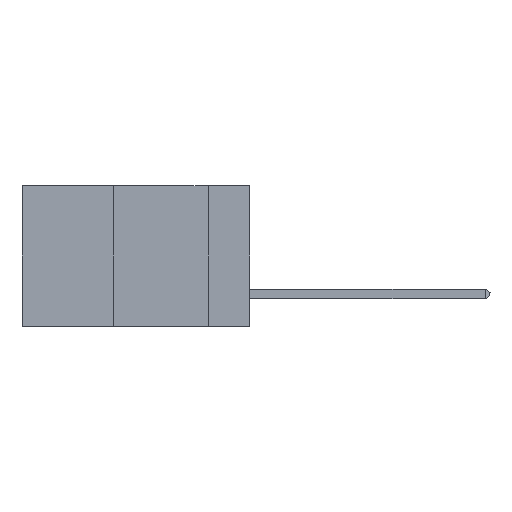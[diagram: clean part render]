
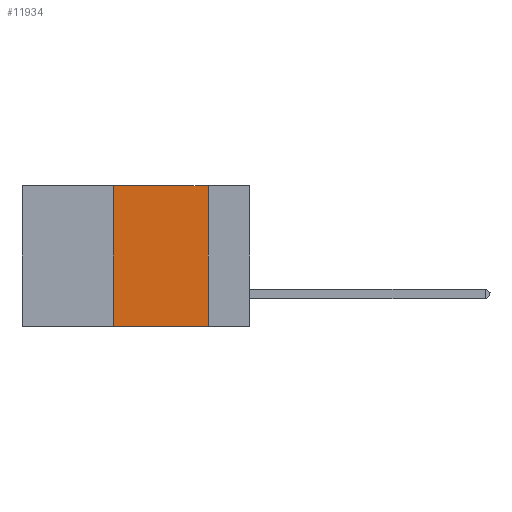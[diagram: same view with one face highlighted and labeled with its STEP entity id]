
A CAD part, left-side view. The second image highlights one B-rep face of the part: STEP entity #11934.
In plain terms, the highlighted planar face has unit normal (-1, 0, 0).
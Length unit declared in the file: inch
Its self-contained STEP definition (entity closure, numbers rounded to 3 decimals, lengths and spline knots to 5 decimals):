
#937 = DIRECTION ( 'NONE',  ( 0., -1., 0. ) ) ;
#1207 = CARTESIAN_POINT ( 'NONE',  ( 0., 0.36, 0. ) ) ;
#2317 = LINE ( 'NONE', #1207, #6592 ) ;
#2643 = ORIENTED_EDGE ( 'NONE', *, *, #22566, .F. ) ;
#4373 = VERTEX_POINT ( 'NONE', #41809 ) ;
#6592 = VECTOR ( 'NONE', #36548, 39.37008 ) ;
#6871 = CARTESIAN_POINT ( 'NONE',  ( 0., 0.11, 0. ) ) ;
#7176 = CARTESIAN_POINT ( 'NONE',  ( 0., 0.11, 0. ) ) ;
#9363 = LINE ( 'NONE', #36799, #19221 ) ;
#11934 = ADVANCED_FACE ( 'NONE', ( #25816 ), #30192, .F. ) ;
#13473 = EDGE_LOOP ( 'NONE', ( #2643, #42642, #21834, #27313 ) ) ;
#16807 = CARTESIAN_POINT ( 'NONE',  ( 0., 0.36, 0. ) ) ;
#18593 = LINE ( 'NONE', #7176, #27817 ) ;
#19221 = VECTOR ( 'NONE', #937, 39.37008 ) ;
#21834 = ORIENTED_EDGE ( 'NONE', *, *, #37795, .F. ) ;
#22566 = EDGE_CURVE ( 'NONE', #31523, #38804, #18593, .T. ) ;
#23443 = VECTOR ( 'NONE', #38262, 39.37008 ) ;
#25108 = AXIS2_PLACEMENT_3D ( 'NONE', #38227, #42205, #30019 ) ;
#25816 = FACE_OUTER_BOUND ( 'NONE', #13473, .T. ) ;
#27313 = ORIENTED_EDGE ( 'NONE', *, *, #47738, .T. ) ;
#27817 = VECTOR ( 'NONE', #34790, 39.37008 ) ;
#30019 = DIRECTION ( 'NONE',  ( 0., 0., -1. ) ) ;
#30192 = PLANE ( 'NONE',  #25108 ) ;
#31523 = VERTEX_POINT ( 'NONE', #6871 ) ;
#34790 = DIRECTION ( 'NONE',  ( 0., 0., -1. ) ) ;
#36548 = DIRECTION ( 'NONE',  ( 0., 0., 1. ) ) ;
#36799 = CARTESIAN_POINT ( 'NONE',  ( 0., 0.6, 0. ) ) ;
#37795 = EDGE_CURVE ( 'NONE', #4373, #50653, #2317, .T. ) ;
#38227 = CARTESIAN_POINT ( 'NONE',  ( 0., 0.6, 0. ) ) ;
#38262 = DIRECTION ( 'NONE',  ( 0., -1., 0. ) ) ;
#38677 = CARTESIAN_POINT ( 'NONE',  ( 0., 0.11, -0.37 ) ) ;
#38804 = VERTEX_POINT ( 'NONE', #38677 ) ;
#41809 = CARTESIAN_POINT ( 'NONE',  ( 0., 0.36, -0.37 ) ) ;
#42205 = DIRECTION ( 'NONE',  ( 1., 0., 0. ) ) ;
#42642 = ORIENTED_EDGE ( 'NONE', *, *, #46831, .F. ) ;
#44890 = LINE ( 'NONE', #50097, #23443 ) ;
#46831 = EDGE_CURVE ( 'NONE', #50653, #31523, #9363, .T. ) ;
#47738 = EDGE_CURVE ( 'NONE', #4373, #38804, #44890, .T. ) ;
#50097 = CARTESIAN_POINT ( 'NONE',  ( 0., 0.6, -0.37 ) ) ;
#50653 = VERTEX_POINT ( 'NONE', #16807 ) ;
